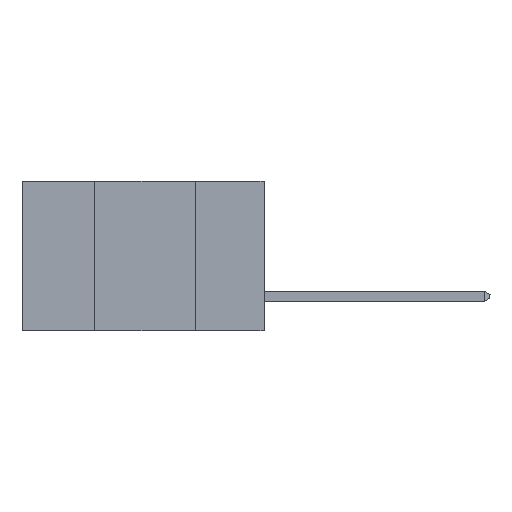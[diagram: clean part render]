
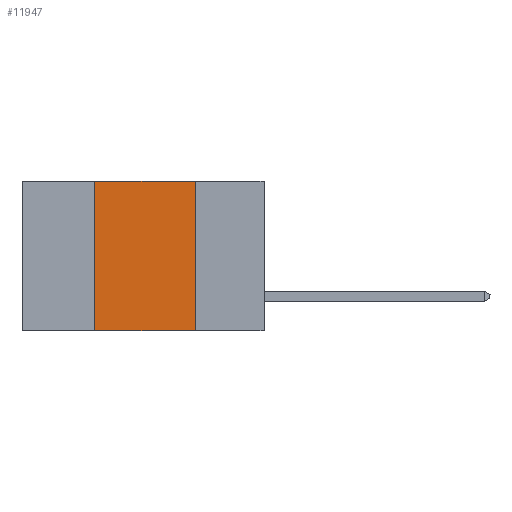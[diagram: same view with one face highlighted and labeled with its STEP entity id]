
A CAD part, left-side view. The second image highlights one B-rep face of the part: STEP entity #11947.
In plain terms, the highlighted planar face has unit normal (-1, 0, 0).
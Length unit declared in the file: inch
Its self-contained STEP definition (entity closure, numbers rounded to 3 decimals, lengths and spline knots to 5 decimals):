
#10 = VERTEX_POINT ( 'NONE', #12058 ) ;
#429 = CARTESIAN_POINT ( 'NONE',  ( 0., 0.6, -0.37 ) ) ;
#532 = DIRECTION ( 'NONE',  ( 0., 0., -1. ) ) ;
#687 = CARTESIAN_POINT ( 'NONE',  ( 0., 0.42, -0.37 ) ) ;
#2506 = EDGE_LOOP ( 'NONE', ( #9340, #6655, #15139, #6242 ) ) ;
#2961 = EDGE_CURVE ( 'NONE', #7124, #11432, #14898, .T. ) ;
#3614 = DIRECTION ( 'NONE',  ( 0., 0., -1. ) ) ;
#4076 = DIRECTION ( 'NONE',  ( 1., 0., 0. ) ) ;
#4860 = EDGE_CURVE ( 'NONE', #11432, #10, #8076, .T. ) ;
#5463 = LINE ( 'NONE', #687, #8061 ) ;
#5606 = VECTOR ( 'NONE', #10898, 39.37008 ) ;
#5923 = CARTESIAN_POINT ( 'NONE',  ( 0., 0.17, -0.37 ) ) ;
#6092 = AXIS2_PLACEMENT_3D ( 'NONE', #10841, #4076, #532 ) ;
#6134 = CARTESIAN_POINT ( 'NONE',  ( 0., 0.42, -0.37 ) ) ;
#6208 = LINE ( 'NONE', #429, #5606 ) ;
#6242 = ORIENTED_EDGE ( 'NONE', *, *, #12286, .T. ) ;
#6655 = ORIENTED_EDGE ( 'NONE', *, *, #2961, .F. ) ;
#7098 = VECTOR ( 'NONE', #3614, 39.37008 ) ;
#7124 = VERTEX_POINT ( 'NONE', #14369 ) ;
#8061 = VECTOR ( 'NONE', #9066, 39.37008 ) ;
#8076 = LINE ( 'NONE', #5923, #7098 ) ;
#9066 = DIRECTION ( 'NONE',  ( 0., 0., 1. ) ) ;
#9340 = ORIENTED_EDGE ( 'NONE', *, *, #4860, .F. ) ;
#10841 = CARTESIAN_POINT ( 'NONE',  ( 0., 0.6, 0. ) ) ;
#10898 = DIRECTION ( 'NONE',  ( 0., -1., 0. ) ) ;
#10997 = VERTEX_POINT ( 'NONE', #6134 ) ;
#11432 = VERTEX_POINT ( 'NONE', #14737 ) ;
#11947 = ADVANCED_FACE ( 'NONE', ( #13159 ), #12319, .F. ) ;
#12022 = EDGE_CURVE ( 'NONE', #10997, #7124, #5463, .T. ) ;
#12058 = CARTESIAN_POINT ( 'NONE',  ( 0., 0.17, -0.37 ) ) ;
#12286 = EDGE_CURVE ( 'NONE', #10997, #10, #6208, .T. ) ;
#12319 = PLANE ( 'NONE',  #6092 ) ;
#12415 = DIRECTION ( 'NONE',  ( 0., -1., 0. ) ) ;
#13159 = FACE_OUTER_BOUND ( 'NONE', #2506, .T. ) ;
#13658 = VECTOR ( 'NONE', #12415, 39.37008 ) ;
#14369 = CARTESIAN_POINT ( 'NONE',  ( 0., 0.42, 0. ) ) ;
#14737 = CARTESIAN_POINT ( 'NONE',  ( 0., 0.17, 0. ) ) ;
#14898 = LINE ( 'NONE', #14967, #13658 ) ;
#14967 = CARTESIAN_POINT ( 'NONE',  ( 0., 0.6, 0. ) ) ;
#15139 = ORIENTED_EDGE ( 'NONE', *, *, #12022, .F. ) ;
